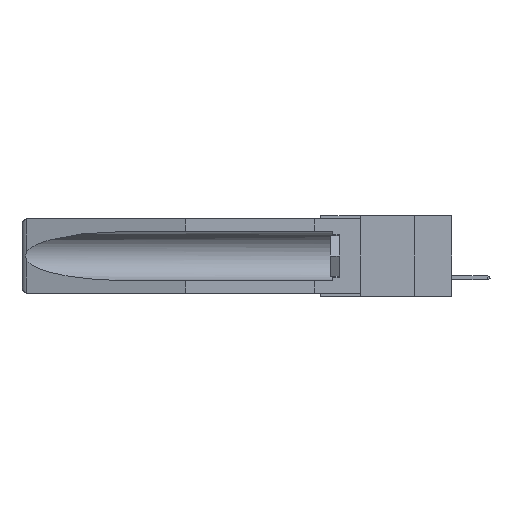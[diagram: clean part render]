
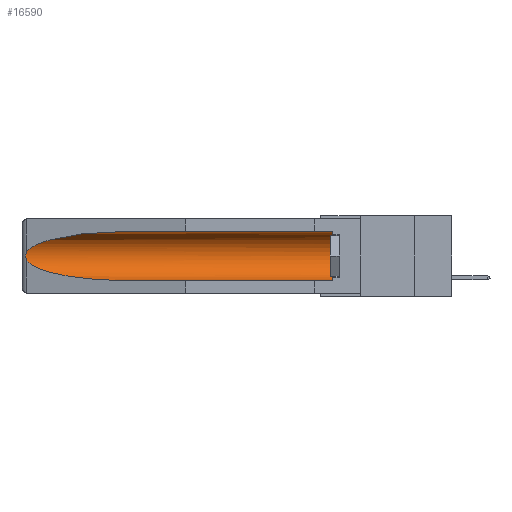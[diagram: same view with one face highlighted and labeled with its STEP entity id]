
A CAD part, left-side view. The second image highlights one B-rep face of the part: STEP entity #16590.
In plain terms, the highlighted cylindrical face has radius 2.857 mm (diameter 5.715 mm), a partial arc.
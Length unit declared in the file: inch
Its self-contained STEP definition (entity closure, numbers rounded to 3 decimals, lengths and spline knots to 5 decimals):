
#343 = DIRECTION ( 'NONE',  ( 0., 1., 0. ) ) ;
#392 = CARTESIAN_POINT ( 'NONE',  ( 0.155, 0.126, -0.059 ) ) ;
#629 = CARTESIAN_POINT ( 'NONE',  ( 0.155, 1.07973, -0.284 ) ) ;
#2416 = LINE ( 'NONE', #5207, #29454 ) ;
#2429 = DIRECTION ( 'NONE',  ( 0., 1., 0. ) ) ;
#2967 = CARTESIAN_POINT ( 'NONE',  ( 0.155, 1.07973, -0.059 ) ) ;
#4450 = CARTESIAN_POINT ( 'NONE',  ( 0.2675, 1.53308, -0.17534 ) ) ;
#4611 = DIRECTION ( 'NONE',  ( 0., 0., 1. ) ) ;
#4725 = ORIENTED_EDGE ( 'NONE', *, *, #27990, .T. ) ;
#5207 = CARTESIAN_POINT ( 'NONE',  ( 0.155, -0.30754, -0.284 ) ) ;
#5740 = DIRECTION ( 'NONE',  ( 0., 0., 1. ) ) ;
#7782 = VERTEX_POINT ( 'NONE', #392 ) ;
#9248 = CARTESIAN_POINT ( 'NONE',  ( 0.155, 0.126, -0.1715 ) ) ;
#9509 = CARTESIAN_POINT ( 'NONE',  ( 0.2675, 1.53308, -0.16763 ) ) ;
#9995 = EDGE_CURVE ( 'NONE', #7782, #26421, #20555, .T. ) ;
#10143 = CIRCLE ( 'NONE', #10843, 0.1125 ) ;
#10563 = CARTESIAN_POINT ( 'NONE',  ( 0.155, 0.126, -0.284 ) ) ;
#10843 = AXIS2_PLACEMENT_3D ( 'NONE', #9248, #14422, #4611 ) ;
#12585 = CARTESIAN_POINT ( 'NONE',  ( 0.155, -0.30754, -0.059 ) ) ;
#13864 = VERTEX_POINT ( 'NONE', #30667 ) ;
#14403 = ORIENTED_EDGE ( 'NONE', *, *, #16378, .F. ) ;
#14422 = DIRECTION ( 'NONE',  ( 0., -1., 0. ) ) ;
#14438 = EDGE_CURVE ( 'NONE', #26421, #29021, #21868, .T. ) ;
#15061 = DIRECTION ( 'NONE',  ( 0., 1., 0. ) ) ;
#15117 = CARTESIAN_POINT ( 'NONE',  ( 0.155, -0.30754, -0.1715 ) ) ;
#15351 = CARTESIAN_POINT ( 'NONE',  ( 0.21114, 1.30732, -0.059 ) ) ;
#15603 = EDGE_CURVE ( 'NONE', #13864, #24277, #21458, .T. ) ;
#16378 = EDGE_CURVE ( 'NONE', #29577, #24277, #2416, .T. ) ;
#16503 = CARTESIAN_POINT ( 'NONE',  ( 0.26654, 1.53092, -0.15636 ) ) ;
#16590 = ADVANCED_FACE ( 'NONE', ( #24048 ), #23643, .F. ) ;
#16932 = CARTESIAN_POINT ( 'NONE',  ( 0.2673, 1.53269, -0.17917 ) ) ;
#17744 = ORIENTED_EDGE ( 'NONE', *, *, #18321, .T. ) ;
#18204 = VECTOR ( 'NONE', #15061, 39.37008 ) ;
#18321 = EDGE_CURVE ( 'NONE', #29021, #13864, #18500, .T. ) ;
#18500 = B_SPLINE_CURVE_WITH_KNOTS ( 'NONE', 3,
 ( #21833, #31800, #16503, #19255, #9509, #4450, #16932, #24130, #24031, #21405 ),
 .UNSPECIFIED., .F., .F.,
 ( 4, 2, 2, 2, 4 ),
 ( 0., 0.00029, 0.00058, 0.00087, 0.00117 ),
 .UNSPECIFIED. ) ;
#18904 = ORIENTED_EDGE ( 'NONE', *, *, #9995, .T. ) ;
#19255 = CARTESIAN_POINT ( 'NONE',  ( 0.2673, 1.5327, -0.16383 ) ) ;
#20555 = LINE ( 'NONE', #12585, #18204 ) ;
#21405 = CARTESIAN_POINT ( 'NONE',  ( 0.26537, 1.52718, -0.19328 ) ) ;
#21458 =( BOUNDED_CURVE ( )  B_SPLINE_CURVE ( 3, ( #25055, #27304, #25372, #629 ),
 .UNSPECIFIED., .F., .F. ) 
 B_SPLINE_CURVE_WITH_KNOTS ( ( 4, 4 ),
 ( 0.1948, 1.5708 ),
 .UNSPECIFIED. ) 
 CURVE ( )  GEOMETRIC_REPRESENTATION_ITEM ( )  RATIONAL_B_SPLINE_CURVE ( ( 1., 0.848, 0.848, 1. ) ) 
 REPRESENTATION_ITEM ( '' )  );
#21833 = CARTESIAN_POINT ( 'NONE',  ( 0.26537, 1.52718, -0.14972 ) ) ;
#21868 =( BOUNDED_CURVE ( )  B_SPLINE_CURVE ( 3, ( #2967, #15351, #25237, #27685 ),
 .UNSPECIFIED., .F., .F. ) 
 B_SPLINE_CURVE_WITH_KNOTS ( ( 4, 4 ),
 ( 4.71239, 6.08839 ),
 .UNSPECIFIED. ) 
 CURVE ( )  GEOMETRIC_REPRESENTATION_ITEM ( )  RATIONAL_B_SPLINE_CURVE ( ( 1., 0.848, 0.848, 1. ) ) 
 REPRESENTATION_ITEM ( '' )  );
#22758 = CARTESIAN_POINT ( 'NONE',  ( 0.155, 1.07973, -0.059 ) ) ;
#23064 = AXIS2_PLACEMENT_3D ( 'NONE', #15117, #343, #5740 ) ;
#23281 = ORIENTED_EDGE ( 'NONE', *, *, #15603, .T. ) ;
#23643 = CYLINDRICAL_SURFACE ( 'NONE', #23064, 0.1125 ) ;
#24031 = CARTESIAN_POINT ( 'NONE',  ( 0.26597, 1.5296, -0.19026 ) ) ;
#24048 = FACE_OUTER_BOUND ( 'NONE', #25364, .T. ) ;
#24130 = CARTESIAN_POINT ( 'NONE',  ( 0.26655, 1.53094, -0.18657 ) ) ;
#24277 = VERTEX_POINT ( 'NONE', #31956 ) ;
#25055 = CARTESIAN_POINT ( 'NONE',  ( 0.26537, 1.52718, -0.19328 ) ) ;
#25237 = CARTESIAN_POINT ( 'NONE',  ( 0.25451, 1.48313, -0.09465 ) ) ;
#25364 = EDGE_LOOP ( 'NONE', ( #27730, #17744, #23281, #14403, #4725, #18904 ) ) ;
#25372 = CARTESIAN_POINT ( 'NONE',  ( 0.21114, 1.30732, -0.284 ) ) ;
#26421 = VERTEX_POINT ( 'NONE', #22758 ) ;
#27304 = CARTESIAN_POINT ( 'NONE',  ( 0.25451, 1.48313, -0.24835 ) ) ;
#27685 = CARTESIAN_POINT ( 'NONE',  ( 0.26537, 1.52718, -0.14972 ) ) ;
#27730 = ORIENTED_EDGE ( 'NONE', *, *, #14438, .T. ) ;
#27889 = CARTESIAN_POINT ( 'NONE',  ( 0.26537, 1.52718, -0.14972 ) ) ;
#27990 = EDGE_CURVE ( 'NONE', #29577, #7782, #10143, .T. ) ;
#29021 = VERTEX_POINT ( 'NONE', #27889 ) ;
#29454 = VECTOR ( 'NONE', #2429, 39.37008 ) ;
#29577 = VERTEX_POINT ( 'NONE', #10563 ) ;
#30667 = CARTESIAN_POINT ( 'NONE',  ( 0.26537, 1.52718, -0.19328 ) ) ;
#31800 = CARTESIAN_POINT ( 'NONE',  ( 0.26597, 1.52961, -0.15275 ) ) ;
#31956 = CARTESIAN_POINT ( 'NONE',  ( 0.155, 1.07973, -0.284 ) ) ;
